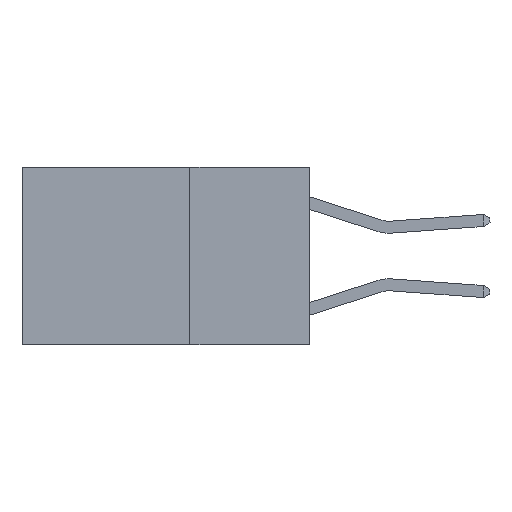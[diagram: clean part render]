
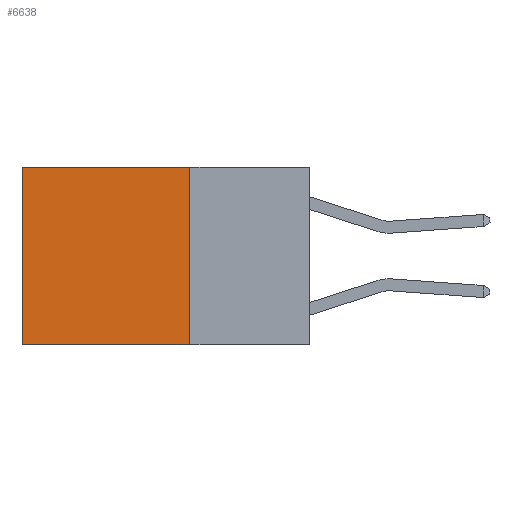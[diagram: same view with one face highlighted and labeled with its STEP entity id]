
A CAD part, left-side view. The second image highlights one B-rep face of the part: STEP entity #6638.
In plain terms, the highlighted planar face has unit normal (-1, 0, 0).
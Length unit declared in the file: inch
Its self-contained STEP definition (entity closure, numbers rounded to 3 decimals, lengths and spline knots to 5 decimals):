
#887 = VECTOR ( 'NONE', #23198, 39.37008 ) ;
#1127 = EDGE_CURVE ( 'NONE', #8522, #3436, #17603, .T. ) ;
#1334 = CARTESIAN_POINT ( 'NONE',  ( 0.2625, 0.6, 0. ) ) ;
#3366 = DIRECTION ( 'NONE',  ( 0., 0., -1. ) ) ;
#3436 = VERTEX_POINT ( 'NONE', #15422 ) ;
#3534 = CARTESIAN_POINT ( 'NONE',  ( 0.2625, 0.6, 0. ) ) ;
#3636 = ORIENTED_EDGE ( 'NONE', *, *, #4068, .T. ) ;
#3649 = DIRECTION ( 'NONE',  ( 1., 0., 0. ) ) ;
#3862 = DIRECTION ( 'NONE',  ( 0., 1., 0. ) ) ;
#4068 = EDGE_CURVE ( 'NONE', #6629, #3436, #20100, .T. ) ;
#4834 = CARTESIAN_POINT ( 'NONE',  ( 0.2625, 0.25, 0. ) ) ;
#5922 = VECTOR ( 'NONE', #3862, 39.37008 ) ;
#6629 = VERTEX_POINT ( 'NONE', #1334 ) ;
#6638 = ADVANCED_FACE ( 'NONE', ( #13816 ), #8849, .F. ) ;
#6899 = AXIS2_PLACEMENT_3D ( 'NONE', #13197, #3649, #13040 ) ;
#7315 = CARTESIAN_POINT ( 'NONE',  ( 0.2625, 0.25, -0.37 ) ) ;
#7434 = CARTESIAN_POINT ( 'NONE',  ( 0.2625, 0.25, 0. ) ) ;
#7522 = CARTESIAN_POINT ( 'NONE',  ( 0.2625, 0.25, -0.37 ) ) ;
#8522 = VERTEX_POINT ( 'NONE', #7315 ) ;
#8849 = PLANE ( 'NONE',  #6899 ) ;
#9346 = VECTOR ( 'NONE', #3366, 39.37008 ) ;
#9587 = ORIENTED_EDGE ( 'NONE', *, *, #21584, .F. ) ;
#11326 = EDGE_LOOP ( 'NONE', ( #3636, #13595, #9587, #20695 ) ) ;
#12349 = VERTEX_POINT ( 'NONE', #12742 ) ;
#12742 = CARTESIAN_POINT ( 'NONE',  ( 0.2625, 0.25, 0. ) ) ;
#12818 = EDGE_CURVE ( 'NONE', #12349, #6629, #19758, .T. ) ;
#13040 = DIRECTION ( 'NONE',  ( 0., 0., -1. ) ) ;
#13083 = VECTOR ( 'NONE', #21683, 39.37008 ) ;
#13197 = CARTESIAN_POINT ( 'NONE',  ( 0.2625, 0.25, 0. ) ) ;
#13595 = ORIENTED_EDGE ( 'NONE', *, *, #1127, .F. ) ;
#13816 = FACE_OUTER_BOUND ( 'NONE', #11326, .T. ) ;
#15422 = CARTESIAN_POINT ( 'NONE',  ( 0.2625, 0.6, -0.37 ) ) ;
#15909 = LINE ( 'NONE', #4834, #887 ) ;
#17603 = LINE ( 'NONE', #7522, #13083 ) ;
#19758 = LINE ( 'NONE', #7434, #5922 ) ;
#20100 = LINE ( 'NONE', #3534, #9346 ) ;
#20695 = ORIENTED_EDGE ( 'NONE', *, *, #12818, .T. ) ;
#21584 = EDGE_CURVE ( 'NONE', #12349, #8522, #15909, .T. ) ;
#21683 = DIRECTION ( 'NONE',  ( 0., 1., 0. ) ) ;
#23198 = DIRECTION ( 'NONE',  ( 0., 0., -1. ) ) ;
